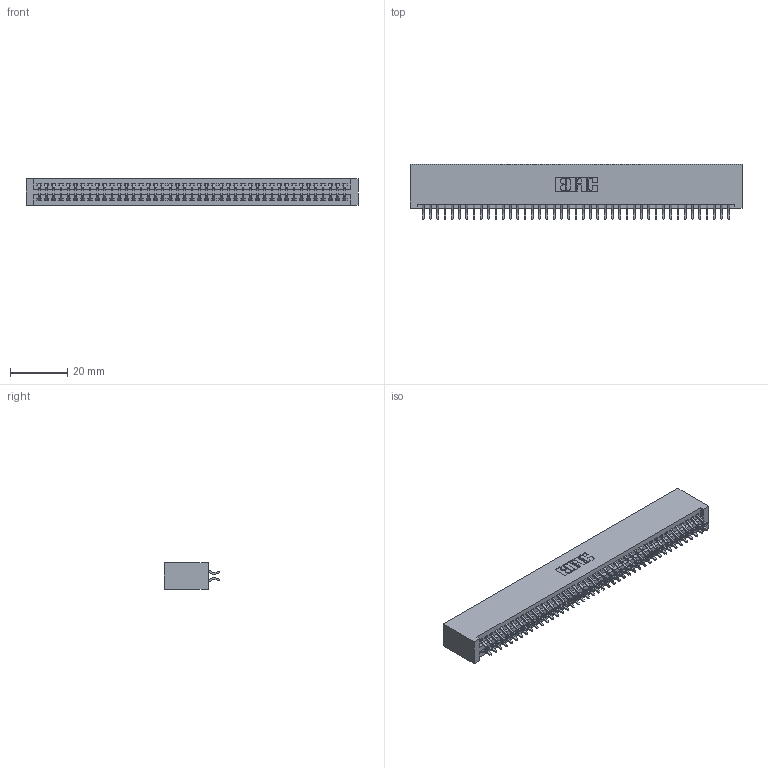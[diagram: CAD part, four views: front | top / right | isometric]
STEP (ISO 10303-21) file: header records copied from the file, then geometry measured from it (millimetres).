
FILE_DESCRIPTION (( 'STEP AP203' ), '1' );
FILE_NAME ('395-086-556-201.STEP', '2018-11-28T21:55:27', ( '' ), ( '' ), 'SwSTEP 2.0', 'SolidWorks 2016', '' );
FILE_SCHEMA (( 'CONFIG_CONTROL_DESIGN' ));
Length unit declared in the file: inch
Products named in the file (3): 345-292-001_556 Tail; 345 Part_No Mounting Lugs; 395-086-556-201
Assembly tree (87 placements, depth 2):
  395-086-556-201
    345 Part_No Mounting Lugs
    345-292-001_556 Tail  x86
Bounding box: 115.82 x 19.24 x 9.4 mm (x, y, z)
Volume: 11873 mm3; surface area: 17797.7 mm2
Topology: 87 solids, 87 shells, 4934 faces, 14679 edges, 9670 vertices
Faces by surface type: plane 3258, cylinder 1676
Entity records: 33547 total; most frequent: CARTESIAN_POINT 5636, ORIENTED_EDGE 5558, DIRECTION 4951, EDGE_CURVE 2779, VECTOR 2475, LINE 2475, VERTEX_POINT 1850, AXIS2_PLACEMENT_3D 1238
